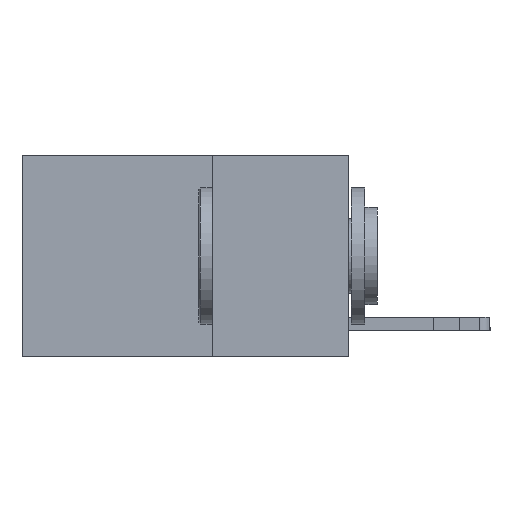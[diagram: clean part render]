
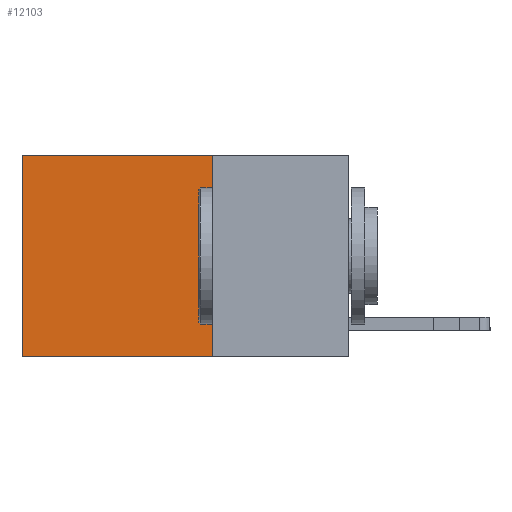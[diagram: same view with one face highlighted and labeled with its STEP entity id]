
A CAD part, left-side view. The second image highlights one B-rep face of the part: STEP entity #12103.
In plain terms, the highlighted planar face has unit normal (-1, 0, 0).
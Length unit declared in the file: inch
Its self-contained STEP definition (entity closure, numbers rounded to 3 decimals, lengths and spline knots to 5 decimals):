
#546 = CARTESIAN_POINT ( 'NONE',  ( 0.2625, 0.25, -0.37 ) ) ;
#1175 = ORIENTED_EDGE ( 'NONE', *, *, #17628, .T. ) ;
#2080 = VECTOR ( 'NONE', #5702, 39.37008 ) ;
#3866 = EDGE_LOOP ( 'NONE', ( #8146, #7825, #13317, #1175 ) ) ;
#4423 = LINE ( 'NONE', #13999, #2080 ) ;
#5702 = DIRECTION ( 'NONE',  ( 0., 0., -1. ) ) ;
#5710 = DIRECTION ( 'NONE',  ( 1., 0., 0. ) ) ;
#5731 = DIRECTION ( 'NONE',  ( 0., 1., 0. ) ) ;
#5888 = EDGE_CURVE ( 'NONE', #19106, #7347, #4423, .T. ) ;
#6520 = EDGE_CURVE ( 'NONE', #16778, #7195, #13225, .T. ) ;
#7188 = LINE ( 'NONE', #15089, #10723 ) ;
#7195 = VERTEX_POINT ( 'NONE', #546 ) ;
#7347 = VERTEX_POINT ( 'NONE', #9660 ) ;
#7379 = DIRECTION ( 'NONE',  ( 0., 0., -1. ) ) ;
#7825 = ORIENTED_EDGE ( 'NONE', *, *, #10448, .F. ) ;
#7840 = VECTOR ( 'NONE', #19754, 39.37008 ) ;
#8049 = CARTESIAN_POINT ( 'NONE',  ( 0.2625, 0.6, 0. ) ) ;
#8146 = ORIENTED_EDGE ( 'NONE', *, *, #5888, .T. ) ;
#8381 = DIRECTION ( 'NONE',  ( 0., 1., 0. ) ) ;
#8470 = CARTESIAN_POINT ( 'NONE',  ( 0.2625, 0.25, 0. ) ) ;
#9660 = CARTESIAN_POINT ( 'NONE',  ( 0.2625, 0.6, -0.37 ) ) ;
#10421 = CARTESIAN_POINT ( 'NONE',  ( 0.2625, 0.25, 0. ) ) ;
#10448 = EDGE_CURVE ( 'NONE', #7195, #7347, #7188, .T. ) ;
#10723 = VECTOR ( 'NONE', #5731, 39.37008 ) ;
#12103 = ADVANCED_FACE ( 'NONE', ( #13810 ), #16652, .F. ) ;
#12357 = AXIS2_PLACEMENT_3D ( 'NONE', #10421, #5710, #7379 ) ;
#13225 = LINE ( 'NONE', #8470, #7840 ) ;
#13317 = ORIENTED_EDGE ( 'NONE', *, *, #6520, .F. ) ;
#13810 = FACE_OUTER_BOUND ( 'NONE', #3866, .T. ) ;
#13999 = CARTESIAN_POINT ( 'NONE',  ( 0.2625, 0.6, 0. ) ) ;
#15089 = CARTESIAN_POINT ( 'NONE',  ( 0.2625, 0.25, -0.37 ) ) ;
#15862 = VECTOR ( 'NONE', #8381, 39.37008 ) ;
#16393 = LINE ( 'NONE', #19768, #15862 ) ;
#16652 = PLANE ( 'NONE',  #12357 ) ;
#16778 = VERTEX_POINT ( 'NONE', #19053 ) ;
#17628 = EDGE_CURVE ( 'NONE', #16778, #19106, #16393, .T. ) ;
#19053 = CARTESIAN_POINT ( 'NONE',  ( 0.2625, 0.25, 0. ) ) ;
#19106 = VERTEX_POINT ( 'NONE', #8049 ) ;
#19754 = DIRECTION ( 'NONE',  ( 0., 0., -1. ) ) ;
#19768 = CARTESIAN_POINT ( 'NONE',  ( 0.2625, 0.25, 0. ) ) ;
